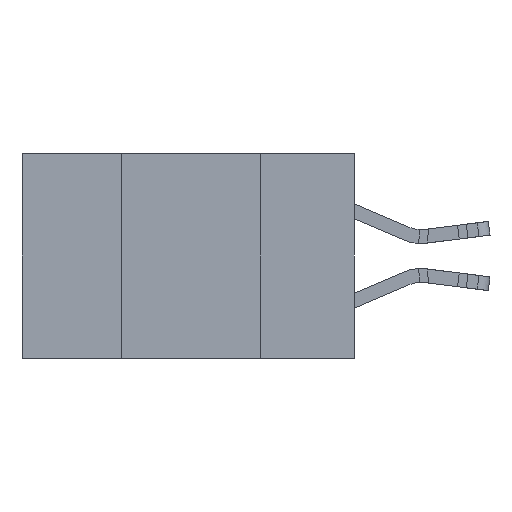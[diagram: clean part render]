
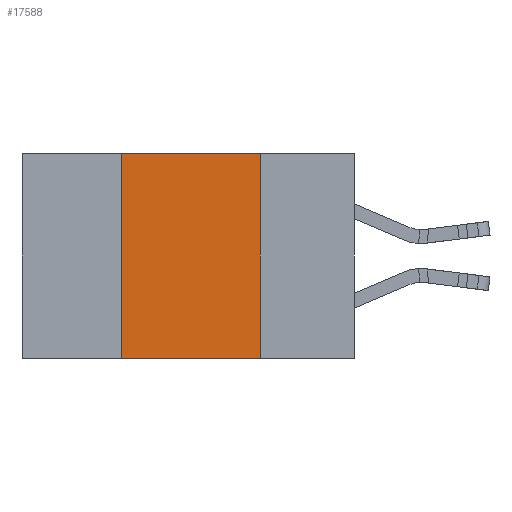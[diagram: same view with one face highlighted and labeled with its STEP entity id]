
A CAD part, left-side view. The second image highlights one B-rep face of the part: STEP entity #17588.
In plain terms, the highlighted planar face has unit normal (-1, 0, 0).
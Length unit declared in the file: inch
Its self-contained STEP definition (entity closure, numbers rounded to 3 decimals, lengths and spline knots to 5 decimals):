
#843 = CARTESIAN_POINT ( 'NONE',  ( 0., 0.6, -0.37 ) ) ;
#3115 = LINE ( 'NONE', #20147, #29778 ) ;
#3337 = CARTESIAN_POINT ( 'NONE',  ( 0., 0.17, 0. ) ) ;
#3528 = DIRECTION ( 'NONE',  ( 0., -1., 0. ) ) ;
#6510 = VECTOR ( 'NONE', #30491, 39.37008 ) ;
#6769 = VERTEX_POINT ( 'NONE', #3337 ) ;
#6913 = VECTOR ( 'NONE', #3528, 39.37008 ) ;
#8958 = CARTESIAN_POINT ( 'NONE',  ( 0., 0.6, 0. ) ) ;
#9316 = VECTOR ( 'NONE', #21810, 39.37008 ) ;
#9369 = CARTESIAN_POINT ( 'NONE',  ( 0., 0.42, 0. ) ) ;
#9647 = EDGE_CURVE ( 'NONE', #27529, #6769, #3115, .T. ) ;
#10942 = EDGE_LOOP ( 'NONE', ( #21697, #19109, #11592, #20659 ) ) ;
#11547 = DIRECTION ( 'NONE',  ( 0., 0., -1. ) ) ;
#11592 = ORIENTED_EDGE ( 'NONE', *, *, #24483, .F. ) ;
#12377 = EDGE_CURVE ( 'NONE', #22354, #17981, #22433, .T. ) ;
#13029 = CARTESIAN_POINT ( 'NONE',  ( 0., 0.17, -0.37 ) ) ;
#15405 = CARTESIAN_POINT ( 'NONE',  ( 0., 0.42, 0. ) ) ;
#16233 = LINE ( 'NONE', #31783, #9316 ) ;
#17588 = ADVANCED_FACE ( 'NONE', ( #22508 ), #19307, .F. ) ;
#17981 = VERTEX_POINT ( 'NONE', #13029 ) ;
#19109 = ORIENTED_EDGE ( 'NONE', *, *, #9647, .F. ) ;
#19307 = PLANE ( 'NONE',  #23478 ) ;
#20147 = CARTESIAN_POINT ( 'NONE',  ( 0., 0.6, 0. ) ) ;
#20651 = EDGE_CURVE ( 'NONE', #6769, #17981, #16233, .T. ) ;
#20659 = ORIENTED_EDGE ( 'NONE', *, *, #12377, .T. ) ;
#21249 = LINE ( 'NONE', #15405, #6510 ) ;
#21697 = ORIENTED_EDGE ( 'NONE', *, *, #20651, .F. ) ;
#21810 = DIRECTION ( 'NONE',  ( 0., 0., -1. ) ) ;
#22354 = VERTEX_POINT ( 'NONE', #23034 ) ;
#22433 = LINE ( 'NONE', #843, #6913 ) ;
#22508 = FACE_OUTER_BOUND ( 'NONE', #10942, .T. ) ;
#23034 = CARTESIAN_POINT ( 'NONE',  ( 0., 0.42, -0.37 ) ) ;
#23478 = AXIS2_PLACEMENT_3D ( 'NONE', #8958, #26861, #11547 ) ;
#24483 = EDGE_CURVE ( 'NONE', #22354, #27529, #21249, .T. ) ;
#25220 = DIRECTION ( 'NONE',  ( 0., -1., 0. ) ) ;
#26861 = DIRECTION ( 'NONE',  ( 1., 0., 0. ) ) ;
#27529 = VERTEX_POINT ( 'NONE', #9369 ) ;
#29778 = VECTOR ( 'NONE', #25220, 39.37008 ) ;
#30491 = DIRECTION ( 'NONE',  ( 0., 0., 1. ) ) ;
#31783 = CARTESIAN_POINT ( 'NONE',  ( 0., 0.17, 0. ) ) ;
